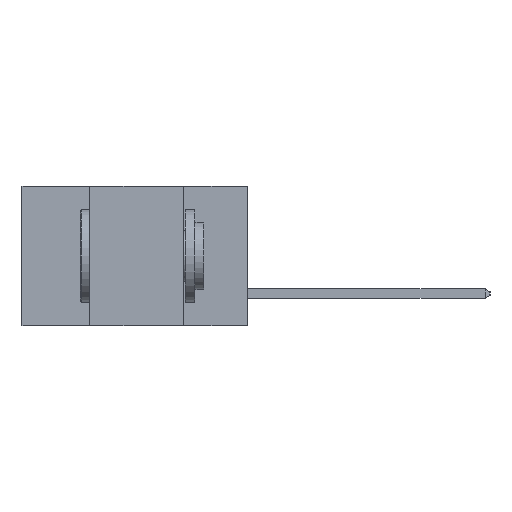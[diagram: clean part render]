
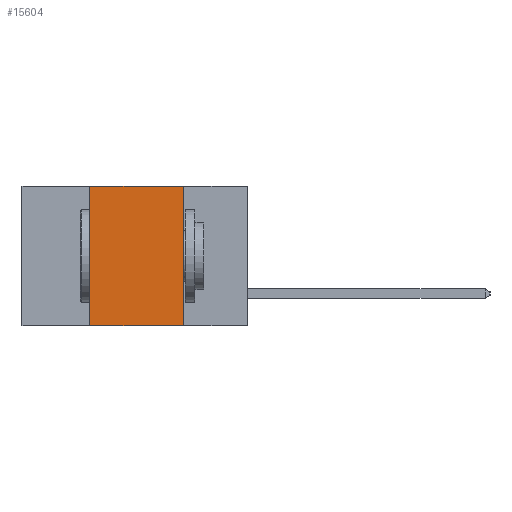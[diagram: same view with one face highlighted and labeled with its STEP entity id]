
A CAD part, left-side view. The second image highlights one B-rep face of the part: STEP entity #15604.
In plain terms, the highlighted planar face has unit normal (-1, 0, 0).
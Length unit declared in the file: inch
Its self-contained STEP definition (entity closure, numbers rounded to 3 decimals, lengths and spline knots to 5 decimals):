
#37 = VERTEX_POINT ( 'NONE', #17695 ) ;
#190 = EDGE_CURVE ( 'NONE', #7055, #37, #5436, .T. ) ;
#1140 = ORIENTED_EDGE ( 'NONE', *, *, #190, .F. ) ;
#1241 = VECTOR ( 'NONE', #15108, 39.37008 ) ;
#1257 = DIRECTION ( 'NONE',  ( 0., -1., 0. ) ) ;
#1381 = ORIENTED_EDGE ( 'NONE', *, *, #18896, .F. ) ;
#1442 = ORIENTED_EDGE ( 'NONE', *, *, #17800, .F. ) ;
#1910 = ORIENTED_EDGE ( 'NONE', *, *, #14541, .T. ) ;
#2502 = CARTESIAN_POINT ( 'NONE',  ( 0., 0.42, -0.37 ) ) ;
#4111 = CARTESIAN_POINT ( 'NONE',  ( 0., 0.17, 0. ) ) ;
#5425 = VECTOR ( 'NONE', #11288, 39.37008 ) ;
#5436 = LINE ( 'NONE', #7189, #1241 ) ;
#5953 = CARTESIAN_POINT ( 'NONE',  ( 0., 0.6, -0.37 ) ) ;
#6517 = CARTESIAN_POINT ( 'NONE',  ( 0., 0.42, 0. ) ) ;
#7055 = VERTEX_POINT ( 'NONE', #4111 ) ;
#7189 = CARTESIAN_POINT ( 'NONE',  ( 0., 0.17, -0.37 ) ) ;
#7210 = EDGE_LOOP ( 'NONE', ( #1140, #1381, #1442, #1910 ) ) ;
#8655 = VERTEX_POINT ( 'NONE', #6517 ) ;
#9384 = DIRECTION ( 'NONE',  ( 0., 0., -1. ) ) ;
#10179 = CARTESIAN_POINT ( 'NONE',  ( 0., 0.6, 0. ) ) ;
#10345 = VERTEX_POINT ( 'NONE', #2502 ) ;
#11288 = DIRECTION ( 'NONE',  ( 0., 0., 1. ) ) ;
#11825 = DIRECTION ( 'NONE',  ( 0., -1., 0. ) ) ;
#13556 = AXIS2_PLACEMENT_3D ( 'NONE', #17458, #19089, #9384 ) ;
#13570 = FACE_OUTER_BOUND ( 'NONE', #7210, .T. ) ;
#13970 = LINE ( 'NONE', #19354, #5425 ) ;
#14541 = EDGE_CURVE ( 'NONE', #10345, #37, #18488, .T. ) ;
#14686 = VECTOR ( 'NONE', #11825, 39.37008 ) ;
#15108 = DIRECTION ( 'NONE',  ( 0., 0., -1. ) ) ;
#15604 = ADVANCED_FACE ( 'NONE', ( #13570 ), #15836, .F. ) ;
#15836 = PLANE ( 'NONE',  #13556 ) ;
#17458 = CARTESIAN_POINT ( 'NONE',  ( 0., 0.6, 0. ) ) ;
#17695 = CARTESIAN_POINT ( 'NONE',  ( 0., 0.17, -0.37 ) ) ;
#17800 = EDGE_CURVE ( 'NONE', #10345, #8655, #13970, .T. ) ;
#18488 = LINE ( 'NONE', #5953, #18994 ) ;
#18896 = EDGE_CURVE ( 'NONE', #8655, #7055, #19001, .T. ) ;
#18994 = VECTOR ( 'NONE', #1257, 39.37008 ) ;
#19001 = LINE ( 'NONE', #10179, #14686 ) ;
#19089 = DIRECTION ( 'NONE',  ( 1., 0., 0. ) ) ;
#19354 = CARTESIAN_POINT ( 'NONE',  ( 0., 0.42, -0.37 ) ) ;
